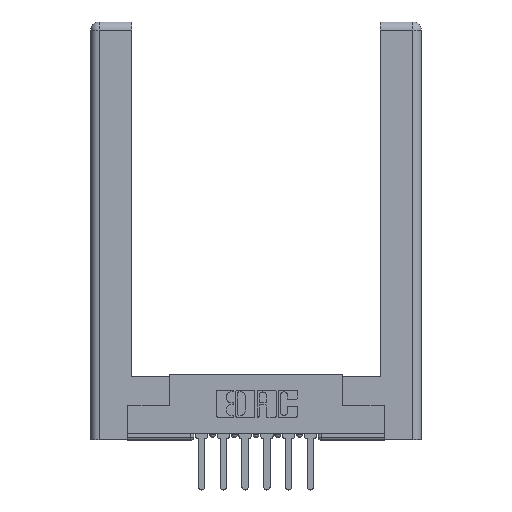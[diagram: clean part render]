
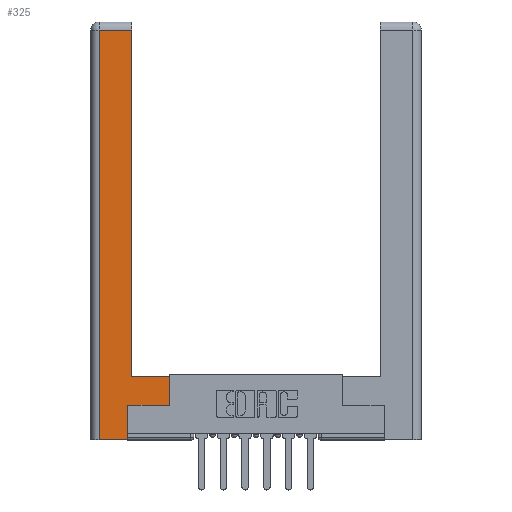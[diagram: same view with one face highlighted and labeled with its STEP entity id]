
A CAD part, top view. The second image highlights one B-rep face of the part: STEP entity #325.
In plain terms, the highlighted planar face has unit normal (0, 0, 1).
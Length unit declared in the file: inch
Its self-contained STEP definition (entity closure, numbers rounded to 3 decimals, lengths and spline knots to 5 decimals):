
#199 = VECTOR ( 'NONE', #10591, 39.37008 ) ;
#325 = ADVANCED_FACE ( 'NONE', ( #10880 ), #6057, .F. ) ;
#348 = EDGE_LOOP ( 'NONE', ( #1705, #5254, #878, #11030, #11706, #6375, #7773, #6727 ) ) ;
#353 = CARTESIAN_POINT ( 'NONE',  ( 0., 0., 0. ) ) ;
#371 = VERTEX_POINT ( 'NONE', #5300 ) ;
#672 = CARTESIAN_POINT ( 'NONE',  ( 0.295, 0.45, 0. ) ) ;
#878 = ORIENTED_EDGE ( 'NONE', *, *, #1573, .T. ) ;
#904 = CARTESIAN_POINT ( 'NONE',  ( 0.295, 0.45, 0. ) ) ;
#927 = VECTOR ( 'NONE', #2342, 39.37008 ) ;
#1086 = LINE ( 'NONE', #8679, #2329 ) ;
#1248 = EDGE_CURVE ( 'NONE', #7812, #4945, #2125, .T. ) ;
#1299 = EDGE_CURVE ( 'NONE', #12258, #11091, #3353, .T. ) ;
#1477 = DIRECTION ( 'NONE',  ( 1., 0., 0. ) ) ;
#1524 = VECTOR ( 'NONE', #8809, 39.37008 ) ;
#1551 = CARTESIAN_POINT ( 'NONE',  ( 0.265, 0.245, 0. ) ) ;
#1573 = EDGE_CURVE ( 'NONE', #371, #7812, #3038, .T. ) ;
#1705 = ORIENTED_EDGE ( 'NONE', *, *, #1299, .T. ) ;
#2065 = CARTESIAN_POINT ( 'NONE',  ( 0.265, 0., 0. ) ) ;
#2125 = LINE ( 'NONE', #2065, #199 ) ;
#2206 = VECTOR ( 'NONE', #3476, 39.37008 ) ;
#2329 = VECTOR ( 'NONE', #10559, 39.37008 ) ;
#2342 = DIRECTION ( 'NONE',  ( 0., -1., 0. ) ) ;
#2839 = DIRECTION ( 'NONE',  ( 0., 1., 0. ) ) ;
#2875 = CARTESIAN_POINT ( 'NONE',  ( 0.565, 0.45, 0. ) ) ;
#3038 = LINE ( 'NONE', #6985, #927 ) ;
#3168 = VECTOR ( 'NONE', #2839, 39.37008 ) ;
#3353 = LINE ( 'NONE', #9591, #2206 ) ;
#3476 = DIRECTION ( 'NONE',  ( 0., 1., 0. ) ) ;
#4234 = CARTESIAN_POINT ( 'NONE',  ( 0.265, 0.245, 0. ) ) ;
#4747 = CARTESIAN_POINT ( 'NONE',  ( 0.295, 2.94, 0. ) ) ;
#4917 = VECTOR ( 'NONE', #1477, 39.37008 ) ;
#4945 = VERTEX_POINT ( 'NONE', #5530 ) ;
#5088 = VERTEX_POINT ( 'NONE', #2875 ) ;
#5184 = LINE ( 'NONE', #6245, #4917 ) ;
#5254 = ORIENTED_EDGE ( 'NONE', *, *, #8688, .T. ) ;
#5300 = CARTESIAN_POINT ( 'NONE',  ( 0.0615, 2.94, 0. ) ) ;
#5530 = CARTESIAN_POINT ( 'NONE',  ( 0.265, 0., 0. ) ) ;
#6057 = PLANE ( 'NONE',  #11270 ) ;
#6236 = DIRECTION ( 'NONE',  ( 0., 1., 0. ) ) ;
#6245 = CARTESIAN_POINT ( 'NONE',  ( 0.565, 0.245, 0. ) ) ;
#6303 = DIRECTION ( 'NONE',  ( -1., 0., 0. ) ) ;
#6375 = ORIENTED_EDGE ( 'NONE', *, *, #6570, .T. ) ;
#6570 = EDGE_CURVE ( 'NONE', #9254, #11770, #5184, .T. ) ;
#6727 = ORIENTED_EDGE ( 'NONE', *, *, #8685, .T. ) ;
#6985 = CARTESIAN_POINT ( 'NONE',  ( 0.0615, 0., 0. ) ) ;
#7658 = CARTESIAN_POINT ( 'NONE',  ( 0.0615, 0., 0. ) ) ;
#7660 = CARTESIAN_POINT ( 'NONE',  ( 0.565, 0.45, 0. ) ) ;
#7773 = ORIENTED_EDGE ( 'NONE', *, *, #10329, .T. ) ;
#7812 = VERTEX_POINT ( 'NONE', #7658 ) ;
#8679 = CARTESIAN_POINT ( 'NONE',  ( 0.0615, 2.94, 0. ) ) ;
#8685 = EDGE_CURVE ( 'NONE', #5088, #12258, #10672, .T. ) ;
#8688 = EDGE_CURVE ( 'NONE', #11091, #371, #1086, .T. ) ;
#8809 = DIRECTION ( 'NONE',  ( -1., 0., 0. ) ) ;
#8916 = CARTESIAN_POINT ( 'NONE',  ( 0.565, 0.245, 0. ) ) ;
#9254 = VERTEX_POINT ( 'NONE', #1551 ) ;
#9361 = VECTOR ( 'NONE', #6236, 39.37008 ) ;
#9591 = CARTESIAN_POINT ( 'NONE',  ( 0.295, 3., 0. ) ) ;
#9615 = EDGE_CURVE ( 'NONE', #4945, #9254, #11769, .T. ) ;
#9669 = LINE ( 'NONE', #7660, #3168 ) ;
#10078 = DIRECTION ( 'NONE',  ( 0., 0., -1. ) ) ;
#10329 = EDGE_CURVE ( 'NONE', #11770, #5088, #9669, .T. ) ;
#10559 = DIRECTION ( 'NONE',  ( -1., 0., 0. ) ) ;
#10591 = DIRECTION ( 'NONE',  ( 1., 0., 0. ) ) ;
#10672 = LINE ( 'NONE', #904, #1524 ) ;
#10880 = FACE_OUTER_BOUND ( 'NONE', #348, .T. ) ;
#11030 = ORIENTED_EDGE ( 'NONE', *, *, #1248, .T. ) ;
#11091 = VERTEX_POINT ( 'NONE', #4747 ) ;
#11270 = AXIS2_PLACEMENT_3D ( 'NONE', #353, #10078, #6303 ) ;
#11706 = ORIENTED_EDGE ( 'NONE', *, *, #9615, .T. ) ;
#11769 = LINE ( 'NONE', #4234, #9361 ) ;
#11770 = VERTEX_POINT ( 'NONE', #8916 ) ;
#12258 = VERTEX_POINT ( 'NONE', #672 ) ;
